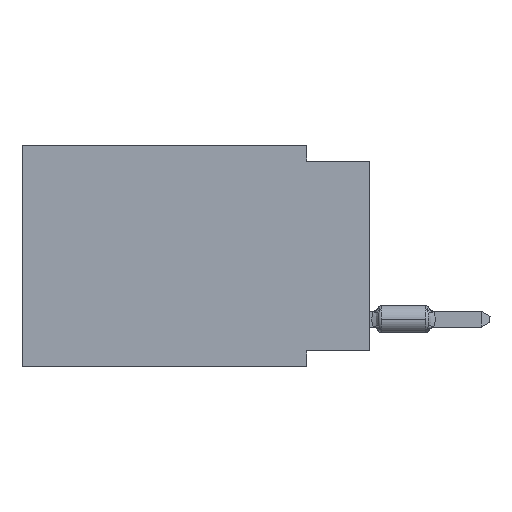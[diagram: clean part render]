
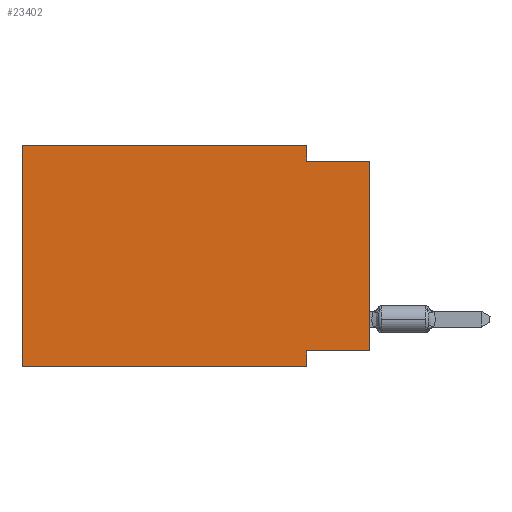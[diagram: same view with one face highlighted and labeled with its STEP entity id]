
A CAD part, left-side view. The second image highlights one B-rep face of the part: STEP entity #23402.
In plain terms, the highlighted planar face has unit normal (-1, 0, 0).
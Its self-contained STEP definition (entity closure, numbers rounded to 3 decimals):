
#570 = ORIENTED_EDGE ( 'NONE', *, *, #19986, .T. ) ;
#650 = ORIENTED_EDGE ( 'NONE', *, *, #1421, .F. ) ;
#716 = CARTESIAN_POINT ( 'NONE',  ( 0., 13.97, -8.89 ) ) ;
#1421 = EDGE_CURVE ( 'NONE', #3881, #22440, #19746, .T. ) ;
#1581 = VECTOR ( 'NONE', #16919, 1000. ) ;
#1942 = ORIENTED_EDGE ( 'NONE', *, *, #4059, .F. ) ;
#3316 = CARTESIAN_POINT ( 'NONE',  ( 0., 2.54, -8.89 ) ) ;
#3696 = VECTOR ( 'NONE', #6630, 1000. ) ;
#3881 = VERTEX_POINT ( 'NONE', #26124 ) ;
#4059 = EDGE_CURVE ( 'NONE', #26102, #16686, #33082, .T. ) ;
#5772 = EDGE_CURVE ( 'NONE', #21745, #22440, #16833, .T. ) ;
#5889 = EDGE_CURVE ( 'NONE', #31152, #3881, #37332, .T. ) ;
#6630 = DIRECTION ( 'NONE',  ( 0., -1., 0. ) ) ;
#7507 = DIRECTION ( 'NONE',  ( 0., 1., 0. ) ) ;
#8060 = CARTESIAN_POINT ( 'NONE',  ( 0., 13.97, 0. ) ) ;
#9019 = DIRECTION ( 'NONE',  ( 0., 0., -1. ) ) ;
#10098 = CARTESIAN_POINT ( 'NONE',  ( 0., 0., -0.635 ) ) ;
#10725 = CARTESIAN_POINT ( 'NONE',  ( 0., 13.97, 0. ) ) ;
#11342 = ORIENTED_EDGE ( 'NONE', *, *, #5772, .T. ) ;
#14396 = CARTESIAN_POINT ( 'NONE',  ( 0., 2.54, -8.89 ) ) ;
#14762 = ORIENTED_EDGE ( 'NONE', *, *, #5889, .F. ) ;
#14895 = VECTOR ( 'NONE', #35955, 1000. ) ;
#16327 = CARTESIAN_POINT ( 'NONE',  ( 0., 0., -8.255 ) ) ;
#16543 = CARTESIAN_POINT ( 'NONE',  ( 0., 0., -8.255 ) ) ;
#16686 = VERTEX_POINT ( 'NONE', #18935 ) ;
#16833 = LINE ( 'NONE', #23813, #39633 ) ;
#16919 = DIRECTION ( 'NONE',  ( 0., -1., 0. ) ) ;
#17221 = ORIENTED_EDGE ( 'NONE', *, *, #18454, .F. ) ;
#17287 = FACE_OUTER_BOUND ( 'NONE', #25615, .T. ) ;
#17319 = CARTESIAN_POINT ( 'NONE',  ( 0., 13.97, 0. ) ) ;
#18136 = ORIENTED_EDGE ( 'NONE', *, *, #35358, .F. ) ;
#18454 = EDGE_CURVE ( 'NONE', #16686, #31152, #32518, .T. ) ;
#18729 = LINE ( 'NONE', #716, #35943 ) ;
#18935 = CARTESIAN_POINT ( 'NONE',  ( 0., 13.97, 0. ) ) ;
#19459 = VECTOR ( 'NONE', #9019, 1000. ) ;
#19509 = CARTESIAN_POINT ( 'NONE',  ( 0., 2.54, -8.255 ) ) ;
#19703 = AXIS2_PLACEMENT_3D ( 'NONE', #8060, #26733, #35761 ) ;
#19746 = LINE ( 'NONE', #10098, #3696 ) ;
#19986 = EDGE_CURVE ( 'NONE', #26102, #28711, #18729, .T. ) ;
#21745 = VERTEX_POINT ( 'NONE', #16327 ) ;
#22204 = CARTESIAN_POINT ( 'NONE',  ( 0., 13.97, -8.89 ) ) ;
#22391 = CARTESIAN_POINT ( 'NONE',  ( 0., 0., -0.635 ) ) ;
#22440 = VERTEX_POINT ( 'NONE', #22391 ) ;
#23242 = PLANE ( 'NONE',  #19703 ) ;
#23402 = ADVANCED_FACE ( 'NONE', ( #17287 ), #23242, .F. ) ;
#23813 = CARTESIAN_POINT ( 'NONE',  ( 0., 0., 0. ) ) ;
#24954 = ORIENTED_EDGE ( 'NONE', *, *, #28998, .F. ) ;
#25615 = EDGE_LOOP ( 'NONE', ( #11342, #650, #14762, #17221, #1942, #570, #24954, #18136 ) ) ;
#26102 = VERTEX_POINT ( 'NONE', #22204 ) ;
#26124 = CARTESIAN_POINT ( 'NONE',  ( 0., 2.54, -0.635 ) ) ;
#26454 = CARTESIAN_POINT ( 'NONE',  ( 0., 2.54, 0. ) ) ;
#26733 = DIRECTION ( 'NONE',  ( 1., 0., 0. ) ) ;
#27104 = DIRECTION ( 'NONE',  ( 0., 0., 1. ) ) ;
#28348 = VECTOR ( 'NONE', #7507, 1000. ) ;
#28533 = LINE ( 'NONE', #3316, #39239 ) ;
#28711 = VERTEX_POINT ( 'NONE', #14396 ) ;
#28998 = EDGE_CURVE ( 'NONE', #36218, #28711, #28533, .T. ) ;
#29063 = LINE ( 'NONE', #16543, #28348 ) ;
#31152 = VERTEX_POINT ( 'NONE', #26454 ) ;
#32231 = DIRECTION ( 'NONE',  ( 0., 0., -1. ) ) ;
#32518 = LINE ( 'NONE', #17319, #1581 ) ;
#33082 = LINE ( 'NONE', #10725, #14895 ) ;
#35358 = EDGE_CURVE ( 'NONE', #21745, #36218, #29063, .T. ) ;
#35761 = DIRECTION ( 'NONE',  ( 0., 0., -1. ) ) ;
#35943 = VECTOR ( 'NONE', #38232, 1000. ) ;
#35955 = DIRECTION ( 'NONE',  ( 0., 0., 1. ) ) ;
#36218 = VERTEX_POINT ( 'NONE', #19509 ) ;
#36734 = CARTESIAN_POINT ( 'NONE',  ( 0., 2.54, 0. ) ) ;
#37332 = LINE ( 'NONE', #36734, #19459 ) ;
#38232 = DIRECTION ( 'NONE',  ( 0., -1., 0. ) ) ;
#39239 = VECTOR ( 'NONE', #32231, 1000. ) ;
#39633 = VECTOR ( 'NONE', #27104, 1000. ) ;
